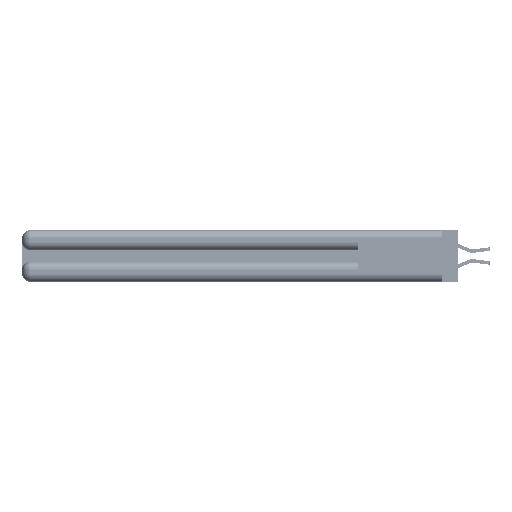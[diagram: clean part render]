
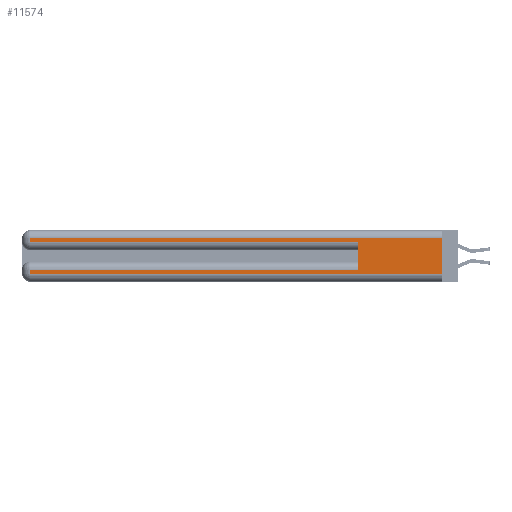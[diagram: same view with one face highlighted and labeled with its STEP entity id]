
A CAD part, left-side view. The second image highlights one B-rep face of the part: STEP entity #11574.
In plain terms, the highlighted planar face has unit normal (-1, 0, 0).
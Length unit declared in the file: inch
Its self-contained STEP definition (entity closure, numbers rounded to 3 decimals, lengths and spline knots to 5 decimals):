
#1062 = CARTESIAN_POINT ( 'NONE',  ( 0., 0., 0.085 ) ) ;
#1658 = VERTEX_POINT ( 'NONE', #43205 ) ;
#3010 = CARTESIAN_POINT ( 'NONE',  ( 0., 2.94, 0.37 ) ) ;
#3864 = EDGE_CURVE ( 'NONE', #32072, #1658, #5258, .T. ) ;
#4841 = DIRECTION ( 'NONE',  ( 0., 1., 0. ) ) ;
#5258 = LINE ( 'NONE', #44291, #32772 ) ;
#7624 = VECTOR ( 'NONE', #30649, 39.37008 ) ;
#8358 = DIRECTION ( 'NONE',  ( 0., -1., 0. ) ) ;
#8808 = ORIENTED_EDGE ( 'NONE', *, *, #20356, .T. ) ;
#9122 = EDGE_CURVE ( 'NONE', #39505, #13450, #40450, .T. ) ;
#9248 = CARTESIAN_POINT ( 'NONE',  ( 0., 0., 0.31 ) ) ;
#9534 = PLANE ( 'NONE',  #16071 ) ;
#9852 = VERTEX_POINT ( 'NONE', #27026 ) ;
#10497 = DIRECTION ( 'NONE',  ( 0., 0., 1. ) ) ;
#11189 = LINE ( 'NONE', #16965, #20397 ) ;
#11450 = LINE ( 'NONE', #11814, #19583 ) ;
#11574 = ADVANCED_FACE ( 'NONE', ( #18792 ), #9534, .F. ) ;
#11814 = CARTESIAN_POINT ( 'NONE',  ( 0., 0., 0.31 ) ) ;
#11951 = ORIENTED_EDGE ( 'NONE', *, *, #16482, .F. ) ;
#13227 = CARTESIAN_POINT ( 'NONE',  ( 0., 0.6, 0.085 ) ) ;
#13450 = VERTEX_POINT ( 'NONE', #41797 ) ;
#13694 = CARTESIAN_POINT ( 'NONE',  ( 0., 2.94, 0.085 ) ) ;
#14691 = LINE ( 'NONE', #1062, #33004 ) ;
#14725 = ORIENTED_EDGE ( 'NONE', *, *, #9122, .T. ) ;
#16071 = AXIS2_PLACEMENT_3D ( 'NONE', #16329, #16479, #40468 ) ;
#16189 = LINE ( 'NONE', #30947, #33415 ) ;
#16329 = CARTESIAN_POINT ( 'NONE',  ( 0., 0., 0.37 ) ) ;
#16479 = DIRECTION ( 'NONE',  ( 1., 0., 0. ) ) ;
#16482 = EDGE_CURVE ( 'NONE', #21473, #1658, #11189, .T. ) ;
#16965 = CARTESIAN_POINT ( 'NONE',  ( 0., 0., 0.37 ) ) ;
#18792 = FACE_OUTER_BOUND ( 'NONE', #31562, .T. ) ;
#19583 = VECTOR ( 'NONE', #4841, 39.37008 ) ;
#20183 = VECTOR ( 'NONE', #10497, 39.37008 ) ;
#20269 = EDGE_CURVE ( 'NONE', #39418, #28103, #14691, .T. ) ;
#20356 = EDGE_CURVE ( 'NONE', #21473, #9852, #11450, .T. ) ;
#20397 = VECTOR ( 'NONE', #34085, 39.37008 ) ;
#20650 = CARTESIAN_POINT ( 'NONE',  ( 0., 2.94, 0.285 ) ) ;
#21197 = ORIENTED_EDGE ( 'NONE', *, *, #20269, .T. ) ;
#21473 = VERTEX_POINT ( 'NONE', #9248 ) ;
#22951 = ORIENTED_EDGE ( 'NONE', *, *, #3864, .T. ) ;
#24624 = ORIENTED_EDGE ( 'NONE', *, *, #40192, .T. ) ;
#25360 = ORIENTED_EDGE ( 'NONE', *, *, #33732, .F. ) ;
#27026 = CARTESIAN_POINT ( 'NONE',  ( 0., 2.94, 0.31 ) ) ;
#27053 = LINE ( 'NONE', #3010, #7624 ) ;
#28103 = VERTEX_POINT ( 'NONE', #13694 ) ;
#28237 = LINE ( 'NONE', #31141, #20183 ) ;
#28658 = EDGE_CURVE ( 'NONE', #28103, #32072, #27053, .T. ) ;
#30649 = DIRECTION ( 'NONE',  ( 0., 0., -1. ) ) ;
#30947 = CARTESIAN_POINT ( 'NONE',  ( 0., 2.94, 0.37 ) ) ;
#31141 = CARTESIAN_POINT ( 'NONE',  ( 0., 0.6, 0.145 ) ) ;
#31562 = EDGE_LOOP ( 'NONE', ( #11951, #8808, #24624, #14725, #25360, #21197, #34792, #22951 ) ) ;
#32072 = VERTEX_POINT ( 'NONE', #35166 ) ;
#32772 = VECTOR ( 'NONE', #34062, 39.37008 ) ;
#33004 = VECTOR ( 'NONE', #38845, 39.37008 ) ;
#33415 = VECTOR ( 'NONE', #34356, 39.37008 ) ;
#33732 = EDGE_CURVE ( 'NONE', #39418, #13450, #28237, .T. ) ;
#34062 = DIRECTION ( 'NONE',  ( 0., -1., 0. ) ) ;
#34085 = DIRECTION ( 'NONE',  ( 0., 0., -1. ) ) ;
#34356 = DIRECTION ( 'NONE',  ( 0., 0., -1. ) ) ;
#34792 = ORIENTED_EDGE ( 'NONE', *, *, #28658, .T. ) ;
#35166 = CARTESIAN_POINT ( 'NONE',  ( 0., 2.94, 0.06 ) ) ;
#38845 = DIRECTION ( 'NONE',  ( 0., 1., 0. ) ) ;
#39308 = CARTESIAN_POINT ( 'NONE',  ( 0., 0., 0.285 ) ) ;
#39418 = VERTEX_POINT ( 'NONE', #13227 ) ;
#39505 = VERTEX_POINT ( 'NONE', #20650 ) ;
#40192 = EDGE_CURVE ( 'NONE', #9852, #39505, #16189, .T. ) ;
#40450 = LINE ( 'NONE', #39308, #41509 ) ;
#40468 = DIRECTION ( 'NONE',  ( 0., 0., -1. ) ) ;
#41509 = VECTOR ( 'NONE', #8358, 39.37008 ) ;
#41797 = CARTESIAN_POINT ( 'NONE',  ( 0., 0.6, 0.285 ) ) ;
#43205 = CARTESIAN_POINT ( 'NONE',  ( 0., 0., 0.06 ) ) ;
#44291 = CARTESIAN_POINT ( 'NONE',  ( 0., 0., 0.06 ) ) ;
